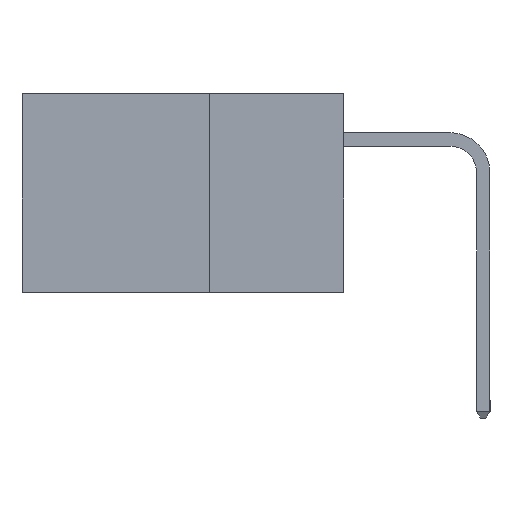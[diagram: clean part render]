
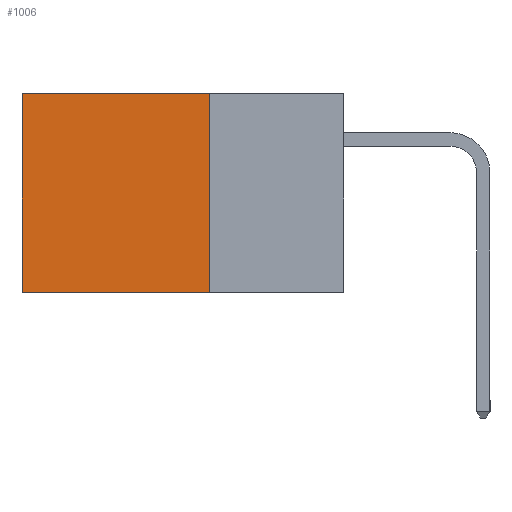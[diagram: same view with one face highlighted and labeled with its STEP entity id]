
A CAD part, left-side view. The second image highlights one B-rep face of the part: STEP entity #1006.
In plain terms, the highlighted planar face has unit normal (-1, 0, 0).
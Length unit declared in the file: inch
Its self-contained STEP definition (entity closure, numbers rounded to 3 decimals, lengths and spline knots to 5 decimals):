
#16 = CARTESIAN_POINT ( 'NONE',  ( 0.2615, 0.25, -0.37 ) ) ;
#208 = VECTOR ( 'NONE', #4828, 39.37008 ) ;
#545 = AXIS2_PLACEMENT_3D ( 'NONE', #16, #8231, #8129 ) ;
#905 = VECTOR ( 'NONE', #7999, 39.37008 ) ;
#1006 = ADVANCED_FACE ( 'NONE', ( #8236 ), #6430, .F. ) ;
#1076 = ORIENTED_EDGE ( 'NONE', *, *, #1938, .T. ) ;
#1090 = ORIENTED_EDGE ( 'NONE', *, *, #8413, .F. ) ;
#1171 = ORIENTED_EDGE ( 'NONE', *, *, #10786, .F. ) ;
#1227 = CARTESIAN_POINT ( 'NONE',  ( 0.2615, 0.25, -0.37 ) ) ;
#1938 = EDGE_CURVE ( 'NONE', #7510, #2185, #8933, .T. ) ;
#2131 = VERTEX_POINT ( 'NONE', #5442 ) ;
#2185 = VERTEX_POINT ( 'NONE', #3365 ) ;
#2444 = CARTESIAN_POINT ( 'NONE',  ( 0.2615, 0.25, -0.37 ) ) ;
#2971 = DIRECTION ( 'NONE',  ( 0., 0., -1. ) ) ;
#3365 = CARTESIAN_POINT ( 'NONE',  ( 0.2615, 0.6, 0. ) ) ;
#4475 = ORIENTED_EDGE ( 'NONE', *, *, #10680, .T. ) ;
#4828 = DIRECTION ( 'NONE',  ( 0., 0., -1. ) ) ;
#5442 = CARTESIAN_POINT ( 'NONE',  ( 0.2615, 0.6, -0.37 ) ) ;
#5597 = LINE ( 'NONE', #7218, #905 ) ;
#5742 = EDGE_LOOP ( 'NONE', ( #4475, #1171, #1090, #1076 ) ) ;
#6430 = PLANE ( 'NONE',  #545 ) ;
#7078 = CARTESIAN_POINT ( 'NONE',  ( 0.2615, 0.6, -0.37 ) ) ;
#7218 = CARTESIAN_POINT ( 'NONE',  ( 0.2615, 0.25, -0.37 ) ) ;
#7420 = LINE ( 'NONE', #1227, #208 ) ;
#7510 = VERTEX_POINT ( 'NONE', #9490 ) ;
#7972 = DIRECTION ( 'NONE',  ( 0., 1., 0. ) ) ;
#7999 = DIRECTION ( 'NONE',  ( 0., 1., 0. ) ) ;
#8057 = CARTESIAN_POINT ( 'NONE',  ( 0.2615, 0.25, 0. ) ) ;
#8129 = DIRECTION ( 'NONE',  ( 0., 0., -1. ) ) ;
#8231 = DIRECTION ( 'NONE',  ( 1., 0., 0. ) ) ;
#8236 = FACE_OUTER_BOUND ( 'NONE', #5742, .T. ) ;
#8413 = EDGE_CURVE ( 'NONE', #7510, #8613, #7420, .T. ) ;
#8613 = VERTEX_POINT ( 'NONE', #2444 ) ;
#8739 = LINE ( 'NONE', #7078, #8968 ) ;
#8933 = LINE ( 'NONE', #8057, #10493 ) ;
#8968 = VECTOR ( 'NONE', #2971, 39.37008 ) ;
#9490 = CARTESIAN_POINT ( 'NONE',  ( 0.2615, 0.25, 0. ) ) ;
#10493 = VECTOR ( 'NONE', #7972, 39.37008 ) ;
#10680 = EDGE_CURVE ( 'NONE', #2185, #2131, #8739, .T. ) ;
#10786 = EDGE_CURVE ( 'NONE', #8613, #2131, #5597, .T. ) ;
